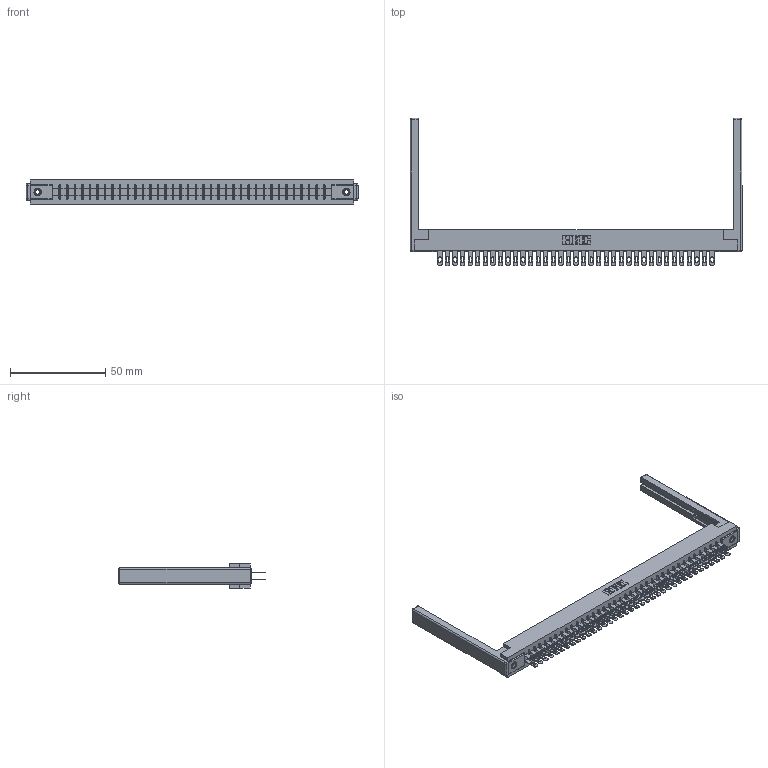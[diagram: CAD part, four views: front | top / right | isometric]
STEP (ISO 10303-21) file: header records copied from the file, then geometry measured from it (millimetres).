
FILE_DESCRIPTION (( 'STEP AP203' ), '1' );
FILE_NAME ('305-074-500-268.STEP', '2019-09-10T06:43:48', ( '' ), ( '' ), 'SwSTEP 2.0', 'SolidWorks 2016', '' );
FILE_SCHEMA (( 'CONFIG_CONTROL_DESIGN' ));
Length unit declared in the file: inch
Products named in the file (5): 307-220-068; 305-290-001_500; 305-074-500-268; 345-250-001_345-250-001-102; 305 Part_.156 Dia
Assembly tree (79 placements, depth 2):
  305-074-500-268
    305 Part_.156 Dia
    305-290-001_500  x74
    345-250-001_345-250-001-102  x2
    307-220-068  x2
Bounding box: 174.04 x 77.14 x 12.7 mm (x, y, z)
Volume: 22738.9 mm3; surface area: 28661.1 mm2
Topology: 79 solids, 79 shells, 3970 faces, 11325 edges, 7330 vertices
Faces by surface type: plane 2228, cylinder 1570, sphere 156, cone 12, torus 4
Entity records: 43451 total; most frequent: CARTESIAN_POINT 7162, ORIENTED_EDGE 7100, DIRECTION 6954, EDGE_CURVE 3550, VECTOR 2854, LINE 2854, VERTEX_POINT 2258, AXIS2_PLACEMENT_3D 2050
